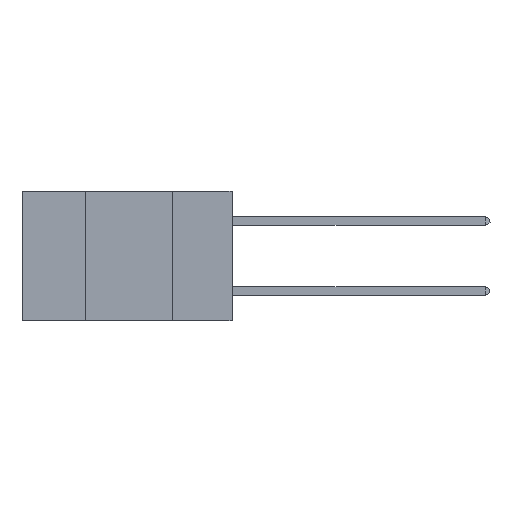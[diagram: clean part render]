
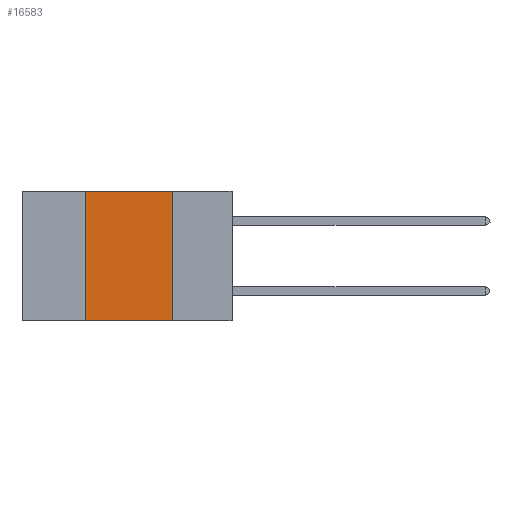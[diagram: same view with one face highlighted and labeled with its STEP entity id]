
A CAD part, left-side view. The second image highlights one B-rep face of the part: STEP entity #16583.
In plain terms, the highlighted planar face has unit normal (-1, 0, 0).
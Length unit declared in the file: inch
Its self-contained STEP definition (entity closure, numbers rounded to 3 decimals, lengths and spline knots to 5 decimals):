
#556 = VECTOR ( 'NONE', #11787, 39.37008 ) ;
#687 = ORIENTED_EDGE ( 'NONE', *, *, #6759, .F. ) ;
#2121 = FACE_OUTER_BOUND ( 'NONE', #17901, .T. ) ;
#2505 = EDGE_CURVE ( 'NONE', #19577, #14970, #6579, .T. ) ;
#3178 = DIRECTION ( 'NONE',  ( 0., 0., 1. ) ) ;
#3846 = VERTEX_POINT ( 'NONE', #14991 ) ;
#4437 = CARTESIAN_POINT ( 'NONE',  ( 0., 0.6, 0. ) ) ;
#5177 = ORIENTED_EDGE ( 'NONE', *, *, #2505, .F. ) ;
#5291 = VERTEX_POINT ( 'NONE', #6585 ) ;
#5474 = ORIENTED_EDGE ( 'NONE', *, *, #11092, .F. ) ;
#6166 = AXIS2_PLACEMENT_3D ( 'NONE', #8142, #16073, #17356 ) ;
#6344 = ORIENTED_EDGE ( 'NONE', *, *, #13262, .T. ) ;
#6579 = LINE ( 'NONE', #4437, #556 ) ;
#6585 = CARTESIAN_POINT ( 'NONE',  ( 0., 0.42, -0.37 ) ) ;
#6759 = EDGE_CURVE ( 'NONE', #5291, #19577, #22009, .T. ) ;
#8142 = CARTESIAN_POINT ( 'NONE',  ( 0., 0.6, 0. ) ) ;
#8312 = DIRECTION ( 'NONE',  ( 0., -1., 0. ) ) ;
#11092 = EDGE_CURVE ( 'NONE', #14970, #3846, #21781, .T. ) ;
#11531 = PLANE ( 'NONE',  #6166 ) ;
#11787 = DIRECTION ( 'NONE',  ( 0., -1., 0. ) ) ;
#12868 = DIRECTION ( 'NONE',  ( 0., 0., -1. ) ) ;
#13262 = EDGE_CURVE ( 'NONE', #5291, #3846, #14062, .T. ) ;
#14062 = LINE ( 'NONE', #19289, #17182 ) ;
#14967 = CARTESIAN_POINT ( 'NONE',  ( 0., 0.17, 0. ) ) ;
#14970 = VERTEX_POINT ( 'NONE', #18572 ) ;
#14991 = CARTESIAN_POINT ( 'NONE',  ( 0., 0.17, -0.37 ) ) ;
#16073 = DIRECTION ( 'NONE',  ( 1., 0., 0. ) ) ;
#16583 = ADVANCED_FACE ( 'NONE', ( #2121 ), #11531, .F. ) ;
#17182 = VECTOR ( 'NONE', #8312, 39.37008 ) ;
#17356 = DIRECTION ( 'NONE',  ( 0., 0., -1. ) ) ;
#17901 = EDGE_LOOP ( 'NONE', ( #5474, #5177, #687, #6344 ) ) ;
#18288 = VECTOR ( 'NONE', #3178, 39.37008 ) ;
#18572 = CARTESIAN_POINT ( 'NONE',  ( 0., 0.17, 0. ) ) ;
#19289 = CARTESIAN_POINT ( 'NONE',  ( 0., 0.6, -0.37 ) ) ;
#19417 = CARTESIAN_POINT ( 'NONE',  ( 0., 0.42, 0. ) ) ;
#19577 = VERTEX_POINT ( 'NONE', #22473 ) ;
#21781 = LINE ( 'NONE', #14967, #22940 ) ;
#22009 = LINE ( 'NONE', #19417, #18288 ) ;
#22473 = CARTESIAN_POINT ( 'NONE',  ( 0., 0.42, 0. ) ) ;
#22940 = VECTOR ( 'NONE', #12868, 39.37008 ) ;
